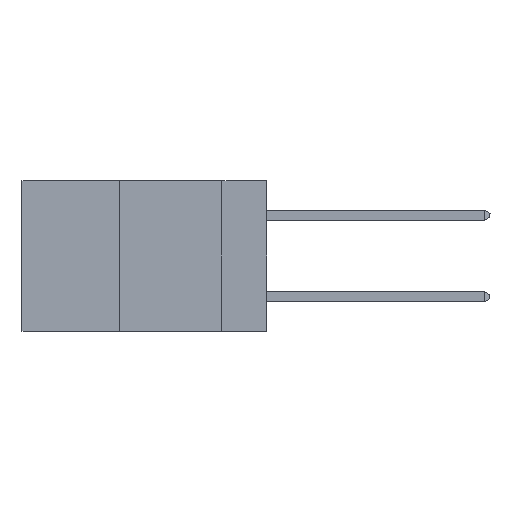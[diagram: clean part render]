
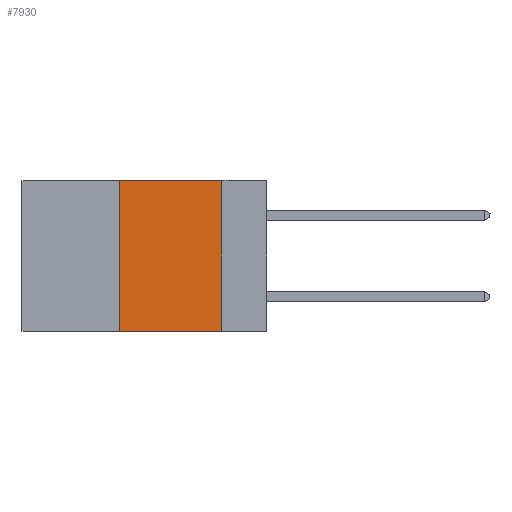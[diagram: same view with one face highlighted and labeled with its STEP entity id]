
A CAD part, left-side view. The second image highlights one B-rep face of the part: STEP entity #7930.
In plain terms, the highlighted planar face has unit normal (-1, 0, 0).
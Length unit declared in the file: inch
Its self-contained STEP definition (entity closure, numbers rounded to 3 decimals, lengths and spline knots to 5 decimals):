
#686 = LINE ( 'NONE', #1383, #3471 ) ;
#764 = CARTESIAN_POINT ( 'NONE',  ( 0., 0.11, 0. ) ) ;
#1383 = CARTESIAN_POINT ( 'NONE',  ( 0., 0.6, 0. ) ) ;
#1451 = DIRECTION ( 'NONE',  ( 0., -1., 0. ) ) ;
#1760 = EDGE_CURVE ( 'NONE', #9376, #8291, #11527, .T. ) ;
#2034 = VECTOR ( 'NONE', #1451, 39.37008 ) ;
#2327 = DIRECTION ( 'NONE',  ( 1., 0., 0. ) ) ;
#2366 = PLANE ( 'NONE',  #2887 ) ;
#2771 = FACE_OUTER_BOUND ( 'NONE', #6731, .T. ) ;
#2887 = AXIS2_PLACEMENT_3D ( 'NONE', #11643, #2327, #4234 ) ;
#3471 = VECTOR ( 'NONE', #9676, 39.37008 ) ;
#3510 = EDGE_CURVE ( 'NONE', #8291, #6666, #686, .T. ) ;
#3532 = DIRECTION ( 'NONE',  ( 0., 0., 1. ) ) ;
#3801 = LINE ( 'NONE', #8133, #2034 ) ;
#4234 = DIRECTION ( 'NONE',  ( 0., 0., -1. ) ) ;
#5248 = VECTOR ( 'NONE', #7322, 39.37008 ) ;
#5588 = CARTESIAN_POINT ( 'NONE',  ( 0., 0.11, 0. ) ) ;
#6322 = CARTESIAN_POINT ( 'NONE',  ( 0., 0.36, 0. ) ) ;
#6666 = VERTEX_POINT ( 'NONE', #5588 ) ;
#6731 = EDGE_LOOP ( 'NONE', ( #8708, #11019, #8400, #7081 ) ) ;
#7081 = ORIENTED_EDGE ( 'NONE', *, *, #10156, .T. ) ;
#7322 = DIRECTION ( 'NONE',  ( 0., 0., -1. ) ) ;
#7930 = ADVANCED_FACE ( 'NONE', ( #2771 ), #2366, .F. ) ;
#8133 = CARTESIAN_POINT ( 'NONE',  ( 0., 0.6, -0.37 ) ) ;
#8291 = VERTEX_POINT ( 'NONE', #8543 ) ;
#8400 = ORIENTED_EDGE ( 'NONE', *, *, #1760, .F. ) ;
#8543 = CARTESIAN_POINT ( 'NONE',  ( 0., 0.36, 0. ) ) ;
#8708 = ORIENTED_EDGE ( 'NONE', *, *, #10417, .F. ) ;
#8860 = CARTESIAN_POINT ( 'NONE',  ( 0., 0.11, -0.37 ) ) ;
#8999 = VECTOR ( 'NONE', #3532, 39.37008 ) ;
#9376 = VERTEX_POINT ( 'NONE', #12008 ) ;
#9676 = DIRECTION ( 'NONE',  ( 0., -1., 0. ) ) ;
#10156 = EDGE_CURVE ( 'NONE', #9376, #11812, #3801, .T. ) ;
#10417 = EDGE_CURVE ( 'NONE', #6666, #11812, #11605, .T. ) ;
#11019 = ORIENTED_EDGE ( 'NONE', *, *, #3510, .F. ) ;
#11527 = LINE ( 'NONE', #6322, #8999 ) ;
#11605 = LINE ( 'NONE', #764, #5248 ) ;
#11643 = CARTESIAN_POINT ( 'NONE',  ( 0., 0.6, 0. ) ) ;
#11812 = VERTEX_POINT ( 'NONE', #8860 ) ;
#12008 = CARTESIAN_POINT ( 'NONE',  ( 0., 0.36, -0.37 ) ) ;
